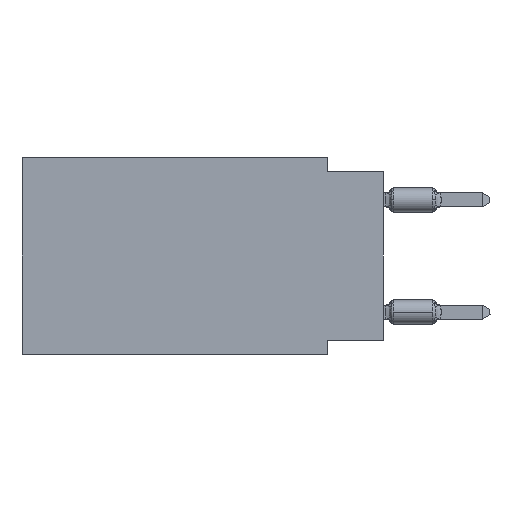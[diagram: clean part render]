
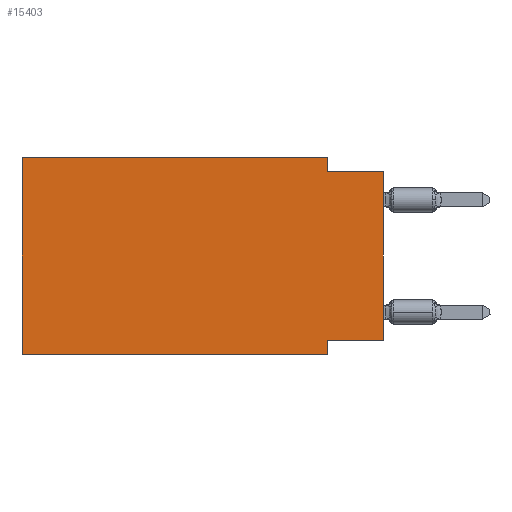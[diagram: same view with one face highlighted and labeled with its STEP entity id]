
A CAD part, left-side view. The second image highlights one B-rep face of the part: STEP entity #15403.
In plain terms, the highlighted planar face has unit normal (-1, 0, 0).
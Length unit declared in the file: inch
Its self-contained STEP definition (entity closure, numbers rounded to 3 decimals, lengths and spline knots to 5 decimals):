
#1449 = DIRECTION ( 'NONE',  ( 0., -1., 0. ) ) ;
#1638 = CARTESIAN_POINT ( 'NONE',  ( 0., 0.1, -0.025 ) ) ;
#2685 = DIRECTION ( 'NONE',  ( 0., 1., 0. ) ) ;
#3983 = EDGE_LOOP ( 'NONE', ( #36696, #22215, #47220, #22196, #44493, #54385, #29300, #51047 ) ) ;
#4072 = LINE ( 'NONE', #45598, #22275 ) ;
#5953 = LINE ( 'NONE', #64855, #67606 ) ;
#6014 = LINE ( 'NONE', #11596, #14315 ) ;
#7587 = LINE ( 'NONE', #65803, #36263 ) ;
#7935 = DIRECTION ( 'NONE',  ( 0., -1., 0. ) ) ;
#9751 = CARTESIAN_POINT ( 'NONE',  ( 0., 0.1, -0.35 ) ) ;
#10987 = EDGE_CURVE ( 'NONE', #44880, #43316, #39517, .T. ) ;
#11501 = VERTEX_POINT ( 'NONE', #63709 ) ;
#11596 = CARTESIAN_POINT ( 'NONE',  ( 0., 0., 0. ) ) ;
#11643 = VERTEX_POINT ( 'NONE', #60523 ) ;
#13936 = VERTEX_POINT ( 'NONE', #56748 ) ;
#14315 = VECTOR ( 'NONE', #54107, 39.37008 ) ;
#14434 = CARTESIAN_POINT ( 'NONE',  ( 0., 0.645, 0. ) ) ;
#15336 = EDGE_CURVE ( 'NONE', #44880, #52478, #7587, .T. ) ;
#15403 = ADVANCED_FACE ( 'NONE', ( #50806 ), #56352, .F. ) ;
#17107 = DIRECTION ( 'NONE',  ( 0., 0., -1. ) ) ;
#18484 = AXIS2_PLACEMENT_3D ( 'NONE', #29201, #50469, #61926 ) ;
#20636 = VECTOR ( 'NONE', #55529, 39.37008 ) ;
#22196 = ORIENTED_EDGE ( 'NONE', *, *, #38349, .F. ) ;
#22215 = ORIENTED_EDGE ( 'NONE', *, *, #68754, .F. ) ;
#22275 = VECTOR ( 'NONE', #2685, 39.37008 ) ;
#29201 = CARTESIAN_POINT ( 'NONE',  ( 0., 0.645, 0. ) ) ;
#29300 = ORIENTED_EDGE ( 'NONE', *, *, #48566, .F. ) ;
#31743 = VECTOR ( 'NONE', #35714, 39.37008 ) ;
#31813 = CARTESIAN_POINT ( 'NONE',  ( 0., 0.1, 0. ) ) ;
#33855 = DIRECTION ( 'NONE',  ( 0., 0., -1. ) ) ;
#35714 = DIRECTION ( 'NONE',  ( 0., -1., 0. ) ) ;
#36263 = VECTOR ( 'NONE', #7935, 39.37008 ) ;
#36575 = VERTEX_POINT ( 'NONE', #1638 ) ;
#36696 = ORIENTED_EDGE ( 'NONE', *, *, #66422, .T. ) ;
#38349 = EDGE_CURVE ( 'NONE', #43316, #40484, #41607, .T. ) ;
#39517 = LINE ( 'NONE', #65980, #20636 ) ;
#40484 = VERTEX_POINT ( 'NONE', #31813 ) ;
#41607 = LINE ( 'NONE', #14434, #31743 ) ;
#42369 = VECTOR ( 'NONE', #1449, 39.37008 ) ;
#43316 = VERTEX_POINT ( 'NONE', #53655 ) ;
#43629 = LINE ( 'NONE', #64864, #46665 ) ;
#44493 = ORIENTED_EDGE ( 'NONE', *, *, #10987, .F. ) ;
#44880 = VERTEX_POINT ( 'NONE', #54615 ) ;
#45038 = CARTESIAN_POINT ( 'NONE',  ( 0., 0., -0.025 ) ) ;
#45598 = CARTESIAN_POINT ( 'NONE',  ( 0., 0., -0.325 ) ) ;
#46665 = VECTOR ( 'NONE', #17107, 39.37008 ) ;
#47220 = ORIENTED_EDGE ( 'NONE', *, *, #52227, .F. ) ;
#48566 = EDGE_CURVE ( 'NONE', #13936, #52478, #43629, .T. ) ;
#49935 = LINE ( 'NONE', #45038, #42369 ) ;
#50469 = DIRECTION ( 'NONE',  ( 1., 0., 0. ) ) ;
#50806 = FACE_OUTER_BOUND ( 'NONE', #3983, .T. ) ;
#51047 = ORIENTED_EDGE ( 'NONE', *, *, #55151, .F. ) ;
#52227 = EDGE_CURVE ( 'NONE', #40484, #36575, #5953, .T. ) ;
#52478 = VERTEX_POINT ( 'NONE', #9751 ) ;
#53655 = CARTESIAN_POINT ( 'NONE',  ( 0., 0.645, 0. ) ) ;
#54107 = DIRECTION ( 'NONE',  ( 0., 0., 1. ) ) ;
#54385 = ORIENTED_EDGE ( 'NONE', *, *, #15336, .T. ) ;
#54615 = CARTESIAN_POINT ( 'NONE',  ( 0., 0.645, -0.35 ) ) ;
#55151 = EDGE_CURVE ( 'NONE', #11643, #13936, #4072, .T. ) ;
#55529 = DIRECTION ( 'NONE',  ( 0., 0., 1. ) ) ;
#56352 = PLANE ( 'NONE',  #18484 ) ;
#56748 = CARTESIAN_POINT ( 'NONE',  ( 0., 0.1, -0.325 ) ) ;
#60523 = CARTESIAN_POINT ( 'NONE',  ( 0., 0., -0.325 ) ) ;
#61926 = DIRECTION ( 'NONE',  ( 0., 0., -1. ) ) ;
#63709 = CARTESIAN_POINT ( 'NONE',  ( 0., 0., -0.025 ) ) ;
#64855 = CARTESIAN_POINT ( 'NONE',  ( 0., 0.1, 0. ) ) ;
#64864 = CARTESIAN_POINT ( 'NONE',  ( 0., 0.1, -0.35 ) ) ;
#65803 = CARTESIAN_POINT ( 'NONE',  ( 0., 0.645, -0.35 ) ) ;
#65980 = CARTESIAN_POINT ( 'NONE',  ( 0., 0.645, 0. ) ) ;
#66422 = EDGE_CURVE ( 'NONE', #11643, #11501, #6014, .T. ) ;
#67606 = VECTOR ( 'NONE', #33855, 39.37008 ) ;
#68754 = EDGE_CURVE ( 'NONE', #36575, #11501, #49935, .T. ) ;
